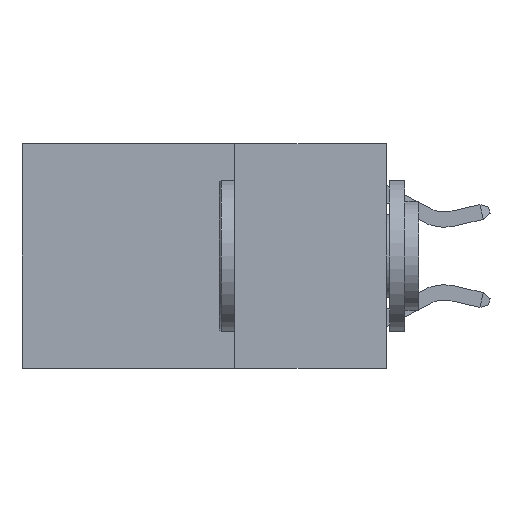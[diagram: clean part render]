
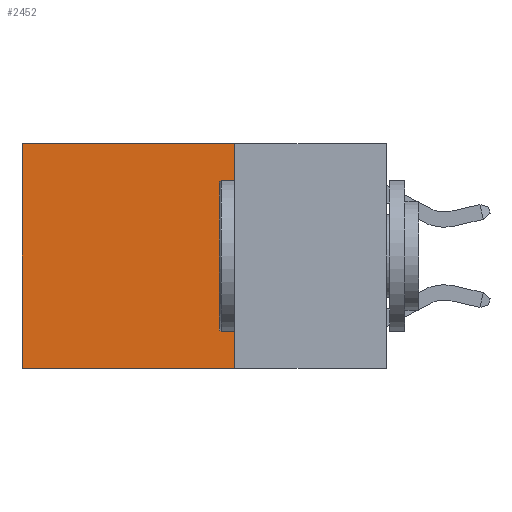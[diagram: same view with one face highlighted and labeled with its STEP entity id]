
A CAD part, left-side view. The second image highlights one B-rep face of the part: STEP entity #2452.
In plain terms, the highlighted planar face has unit normal (-1, 0, 0).
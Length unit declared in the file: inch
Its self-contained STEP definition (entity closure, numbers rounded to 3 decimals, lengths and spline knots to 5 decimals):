
#423 = CARTESIAN_POINT ( 'NONE',  ( 0.2625, 0.25, 0. ) ) ;
#649 = CARTESIAN_POINT ( 'NONE',  ( 0.2625, 0.25, -0.37 ) ) ;
#848 = CARTESIAN_POINT ( 'NONE',  ( 0.2625, 0.6, -0.37 ) ) ;
#1107 = EDGE_CURVE ( 'NONE', #20913, #3162, #20794, .T. ) ;
#1331 = AXIS2_PLACEMENT_3D ( 'NONE', #7004, #16512, #7114 ) ;
#1969 = CARTESIAN_POINT ( 'NONE',  ( 0.2625, 0.6, 0. ) ) ;
#2452 = ADVANCED_FACE ( 'NONE', ( #16904 ), #8766, .F. ) ;
#3162 = VERTEX_POINT ( 'NONE', #848 ) ;
#3180 = VECTOR ( 'NONE', #10336, 39.37008 ) ;
#3545 = CARTESIAN_POINT ( 'NONE',  ( 0.2625, 0.25, 0. ) ) ;
#5376 = VECTOR ( 'NONE', #11067, 39.37008 ) ;
#5618 = VERTEX_POINT ( 'NONE', #13875 ) ;
#5677 = ORIENTED_EDGE ( 'NONE', *, *, #1107, .F. ) ;
#7004 = CARTESIAN_POINT ( 'NONE',  ( 0.2625, 0.25, 0. ) ) ;
#7073 = DIRECTION ( 'NONE',  ( 0., 0., -1. ) ) ;
#7114 = DIRECTION ( 'NONE',  ( 0., 0., -1. ) ) ;
#8239 = EDGE_LOOP ( 'NONE', ( #13112, #5677, #19279, #9559 ) ) ;
#8766 = PLANE ( 'NONE',  #1331 ) ;
#9559 = ORIENTED_EDGE ( 'NONE', *, *, #19873, .T. ) ;
#10230 = EDGE_CURVE ( 'NONE', #5618, #20913, #15356, .T. ) ;
#10336 = DIRECTION ( 'NONE',  ( 0., 0., -1. ) ) ;
#11067 = DIRECTION ( 'NONE',  ( 0., 1., 0. ) ) ;
#12958 = VECTOR ( 'NONE', #15333, 39.37008 ) ;
#13112 = ORIENTED_EDGE ( 'NONE', *, *, #20309, .T. ) ;
#13219 = VERTEX_POINT ( 'NONE', #1969 ) ;
#13875 = CARTESIAN_POINT ( 'NONE',  ( 0.2625, 0.25, 0. ) ) ;
#15333 = DIRECTION ( 'NONE',  ( 0., 1., 0. ) ) ;
#15356 = LINE ( 'NONE', #423, #18336 ) ;
#16512 = DIRECTION ( 'NONE',  ( 1., 0., 0. ) ) ;
#16904 = FACE_OUTER_BOUND ( 'NONE', #8239, .T. ) ;
#17166 = LINE ( 'NONE', #3545, #12958 ) ;
#18336 = VECTOR ( 'NONE', #7073, 39.37008 ) ;
#18365 = LINE ( 'NONE', #19953, #3180 ) ;
#19279 = ORIENTED_EDGE ( 'NONE', *, *, #10230, .F. ) ;
#19873 = EDGE_CURVE ( 'NONE', #5618, #13219, #17166, .T. ) ;
#19953 = CARTESIAN_POINT ( 'NONE',  ( 0.2625, 0.6, 0. ) ) ;
#20309 = EDGE_CURVE ( 'NONE', #13219, #3162, #18365, .T. ) ;
#20794 = LINE ( 'NONE', #21015, #5376 ) ;
#20913 = VERTEX_POINT ( 'NONE', #649 ) ;
#21015 = CARTESIAN_POINT ( 'NONE',  ( 0.2625, 0.25, -0.37 ) ) ;
